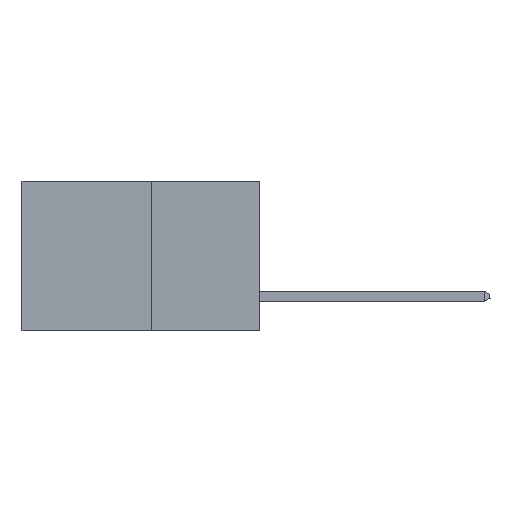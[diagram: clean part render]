
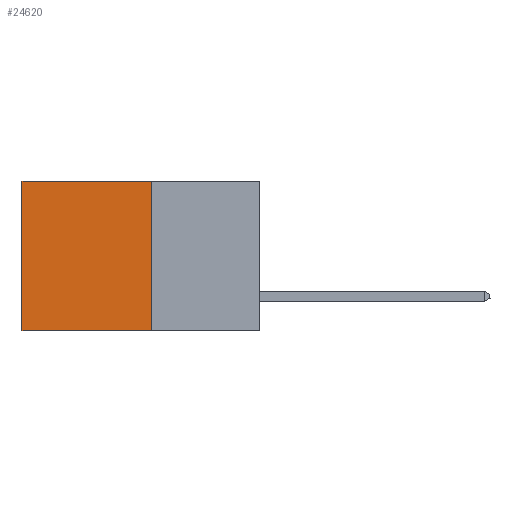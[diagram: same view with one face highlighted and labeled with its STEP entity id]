
A CAD part, left-side view. The second image highlights one B-rep face of the part: STEP entity #24620.
In plain terms, the highlighted planar face has unit normal (-1, 0, 0).
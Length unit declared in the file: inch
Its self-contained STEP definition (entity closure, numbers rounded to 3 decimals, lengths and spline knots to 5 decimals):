
#376 = VERTEX_POINT ( 'NONE', #27558 ) ;
#1261 = ORIENTED_EDGE ( 'NONE', *, *, #3122, .T. ) ;
#2013 = ORIENTED_EDGE ( 'NONE', *, *, #8145, .T. ) ;
#2765 = CARTESIAN_POINT ( 'NONE',  ( 0.277, 0.27, 0. ) ) ;
#3122 = EDGE_CURVE ( 'NONE', #376, #23936, #3288, .T. ) ;
#3272 = LINE ( 'NONE', #21847, #15460 ) ;
#3288 = LINE ( 'NONE', #27797, #14772 ) ;
#6765 = VERTEX_POINT ( 'NONE', #2765 ) ;
#7442 = AXIS2_PLACEMENT_3D ( 'NONE', #28358, #21616, #7942 ) ;
#7750 = ORIENTED_EDGE ( 'NONE', *, *, #23971, .F. ) ;
#7942 = DIRECTION ( 'NONE',  ( 0., 0., -1. ) ) ;
#8145 = EDGE_CURVE ( 'NONE', #6765, #376, #16995, .T. ) ;
#8257 = FACE_OUTER_BOUND ( 'NONE', #21972, .T. ) ;
#9416 = DIRECTION ( 'NONE',  ( 0., 1., 0. ) ) ;
#9895 = VECTOR ( 'NONE', #23566, 39.37008 ) ;
#12281 = EDGE_CURVE ( 'NONE', #6765, #25182, #28029, .T. ) ;
#14772 = VECTOR ( 'NONE', #27900, 39.37008 ) ;
#15460 = VECTOR ( 'NONE', #26301, 39.37008 ) ;
#16995 = LINE ( 'NONE', #23028, #28369 ) ;
#19339 = PLANE ( 'NONE',  #7442 ) ;
#19456 = CARTESIAN_POINT ( 'NONE',  ( 0.277, 0.59, -0.37 ) ) ;
#21103 = CARTESIAN_POINT ( 'NONE',  ( 0.277, 0.27, -0.37 ) ) ;
#21305 = CARTESIAN_POINT ( 'NONE',  ( 0.277, 0.27, -0.37 ) ) ;
#21616 = DIRECTION ( 'NONE',  ( 1., 0., 0. ) ) ;
#21847 = CARTESIAN_POINT ( 'NONE',  ( 0.277, 0.27, -0.37 ) ) ;
#21972 = EDGE_LOOP ( 'NONE', ( #1261, #7750, #23434, #2013 ) ) ;
#23028 = CARTESIAN_POINT ( 'NONE',  ( 0.277, 0.27, 0. ) ) ;
#23434 = ORIENTED_EDGE ( 'NONE', *, *, #12281, .F. ) ;
#23566 = DIRECTION ( 'NONE',  ( 0., 0., -1. ) ) ;
#23936 = VERTEX_POINT ( 'NONE', #19456 ) ;
#23971 = EDGE_CURVE ( 'NONE', #25182, #23936, #3272, .T. ) ;
#24620 = ADVANCED_FACE ( 'NONE', ( #8257 ), #19339, .F. ) ;
#25182 = VERTEX_POINT ( 'NONE', #21103 ) ;
#26301 = DIRECTION ( 'NONE',  ( 0., 1., 0. ) ) ;
#27558 = CARTESIAN_POINT ( 'NONE',  ( 0.277, 0.59, 0. ) ) ;
#27797 = CARTESIAN_POINT ( 'NONE',  ( 0.277, 0.59, -0.37 ) ) ;
#27900 = DIRECTION ( 'NONE',  ( 0., 0., -1. ) ) ;
#28029 = LINE ( 'NONE', #21305, #9895 ) ;
#28358 = CARTESIAN_POINT ( 'NONE',  ( 0.277, 0.27, -0.37 ) ) ;
#28369 = VECTOR ( 'NONE', #9416, 39.37008 ) ;
